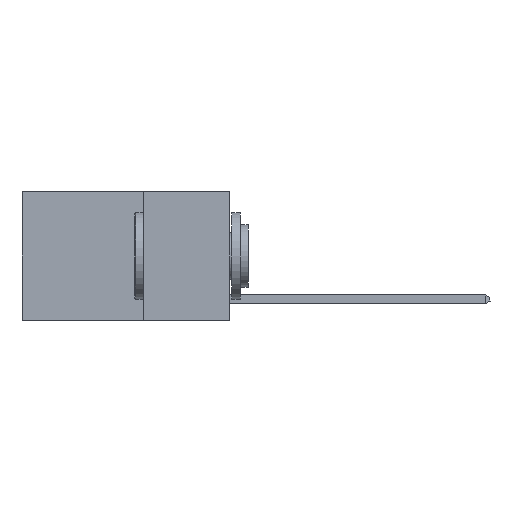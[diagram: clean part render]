
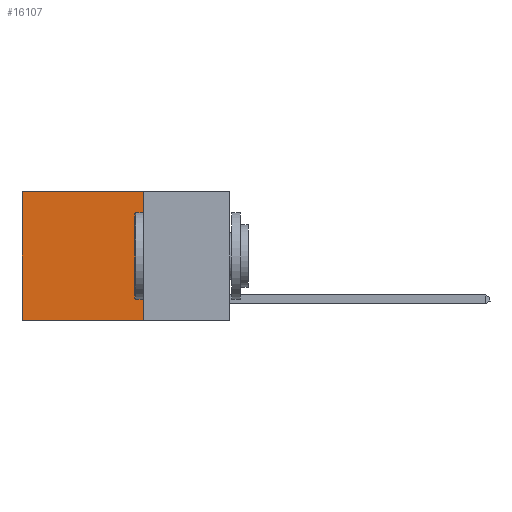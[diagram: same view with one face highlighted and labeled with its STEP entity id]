
A CAD part, left-side view. The second image highlights one B-rep face of the part: STEP entity #16107.
In plain terms, the highlighted planar face has unit normal (-1, 0, 0).
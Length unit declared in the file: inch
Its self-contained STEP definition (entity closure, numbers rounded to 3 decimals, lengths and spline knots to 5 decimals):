
#1190 = DIRECTION ( 'NONE',  ( 0., 0., -1. ) ) ;
#1462 = VECTOR ( 'NONE', #13346, 39.37008 ) ;
#1744 = EDGE_LOOP ( 'NONE', ( #10229, #8998, #5273, #8837 ) ) ;
#2548 = CARTESIAN_POINT ( 'NONE',  ( 0.2625, 0.25, -0.37 ) ) ;
#3873 = EDGE_CURVE ( 'NONE', #7932, #13246, #16407, .T. ) ;
#4012 = CARTESIAN_POINT ( 'NONE',  ( 0.2625, 0.6, -0.37 ) ) ;
#4200 = CARTESIAN_POINT ( 'NONE',  ( 0.2625, 0.25, 0. ) ) ;
#5151 = VERTEX_POINT ( 'NONE', #4012 ) ;
#5273 = ORIENTED_EDGE ( 'NONE', *, *, #18312, .F. ) ;
#5414 = VECTOR ( 'NONE', #5837, 39.37008 ) ;
#5793 = CARTESIAN_POINT ( 'NONE',  ( 0.2625, 0.25, -0.37 ) ) ;
#5837 = DIRECTION ( 'NONE',  ( 0., 0., -1. ) ) ;
#5996 = FACE_OUTER_BOUND ( 'NONE', #1744, .T. ) ;
#7742 = CARTESIAN_POINT ( 'NONE',  ( 0.2625, 0.25, 0. ) ) ;
#7890 = CARTESIAN_POINT ( 'NONE',  ( 0.2625, 0.25, 0. ) ) ;
#7932 = VERTEX_POINT ( 'NONE', #7742 ) ;
#8837 = ORIENTED_EDGE ( 'NONE', *, *, #3873, .T. ) ;
#8998 = ORIENTED_EDGE ( 'NONE', *, *, #16150, .F. ) ;
#9612 = EDGE_CURVE ( 'NONE', #13246, #5151, #16869, .T. ) ;
#10229 = ORIENTED_EDGE ( 'NONE', *, *, #9612, .T. ) ;
#10274 = DIRECTION ( 'NONE',  ( 1., 0., 0. ) ) ;
#11552 = AXIS2_PLACEMENT_3D ( 'NONE', #4200, #10274, #1190 ) ;
#12462 = VECTOR ( 'NONE', #18817, 39.37008 ) ;
#13246 = VERTEX_POINT ( 'NONE', #14265 ) ;
#13346 = DIRECTION ( 'NONE',  ( 0., 1., 0. ) ) ;
#13858 = DIRECTION ( 'NONE',  ( 0., 0., -1. ) ) ;
#13988 = LINE ( 'NONE', #5793, #1462 ) ;
#14165 = VECTOR ( 'NONE', #13858, 39.37008 ) ;
#14265 = CARTESIAN_POINT ( 'NONE',  ( 0.2625, 0.6, 0. ) ) ;
#14629 = LINE ( 'NONE', #7890, #14165 ) ;
#14835 = CARTESIAN_POINT ( 'NONE',  ( 0.2625, 0.6, 0. ) ) ;
#16107 = ADVANCED_FACE ( 'NONE', ( #5996 ), #19156, .F. ) ;
#16150 = EDGE_CURVE ( 'NONE', #17381, #5151, #13988, .T. ) ;
#16407 = LINE ( 'NONE', #17346, #12462 ) ;
#16869 = LINE ( 'NONE', #14835, #5414 ) ;
#17346 = CARTESIAN_POINT ( 'NONE',  ( 0.2625, 0.25, 0. ) ) ;
#17381 = VERTEX_POINT ( 'NONE', #2548 ) ;
#18312 = EDGE_CURVE ( 'NONE', #7932, #17381, #14629, .T. ) ;
#18817 = DIRECTION ( 'NONE',  ( 0., 1., 0. ) ) ;
#19156 = PLANE ( 'NONE',  #11552 ) ;
